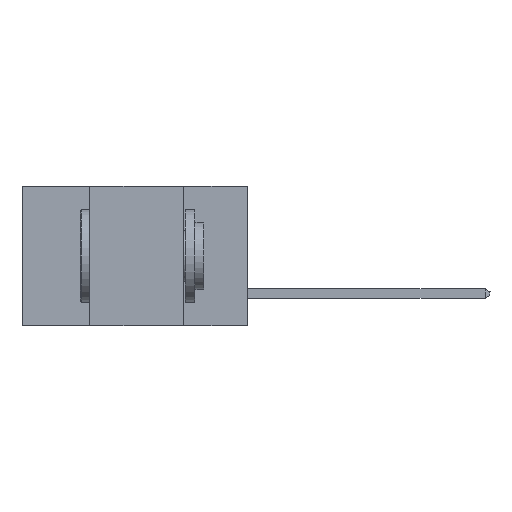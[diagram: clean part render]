
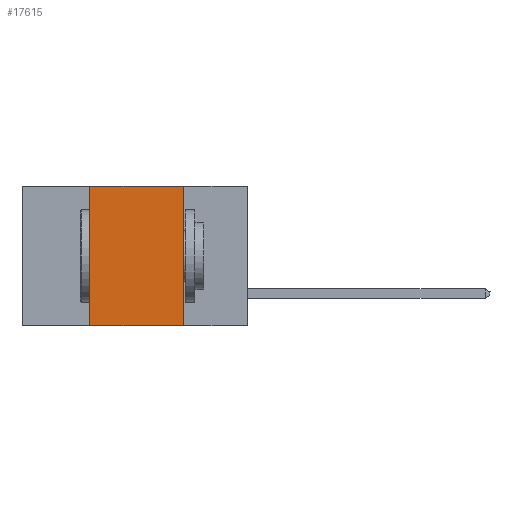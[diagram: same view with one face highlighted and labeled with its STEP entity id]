
A CAD part, left-side view. The second image highlights one B-rep face of the part: STEP entity #17615.
In plain terms, the highlighted planar face has unit normal (-1, 0, 0).
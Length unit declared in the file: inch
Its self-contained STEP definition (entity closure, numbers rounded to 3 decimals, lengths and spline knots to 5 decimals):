
#25 = EDGE_CURVE ( 'NONE', #7448, #22816, #8472, .T. ) ;
#639 = CARTESIAN_POINT ( 'NONE',  ( 0., 0.42, -0.37 ) ) ;
#665 = LINE ( 'NONE', #17799, #3531 ) ;
#713 = CARTESIAN_POINT ( 'NONE',  ( 0., 0.6, 0. ) ) ;
#909 = EDGE_CURVE ( 'NONE', #7448, #4018, #665, .T. ) ;
#1226 = AXIS2_PLACEMENT_3D ( 'NONE', #713, #13991, #21608 ) ;
#1958 = LINE ( 'NONE', #5464, #15267 ) ;
#2379 = CARTESIAN_POINT ( 'NONE',  ( 0., 0.42, -0.37 ) ) ;
#2574 = FACE_OUTER_BOUND ( 'NONE', #11931, .T. ) ;
#3152 = CARTESIAN_POINT ( 'NONE',  ( 0., 0.17, -0.37 ) ) ;
#3415 = CARTESIAN_POINT ( 'NONE',  ( 0., 0.17, 0. ) ) ;
#3531 = VECTOR ( 'NONE', #14071, 39.37008 ) ;
#4018 = VERTEX_POINT ( 'NONE', #16116 ) ;
#5464 = CARTESIAN_POINT ( 'NONE',  ( 0., 0.6, 0. ) ) ;
#7202 = VECTOR ( 'NONE', #12820, 39.37008 ) ;
#7448 = VERTEX_POINT ( 'NONE', #2379 ) ;
#7686 = CARTESIAN_POINT ( 'NONE',  ( 0., 0.42, 0. ) ) ;
#8461 = ORIENTED_EDGE ( 'NONE', *, *, #22922, .F. ) ;
#8472 = LINE ( 'NONE', #639, #16629 ) ;
#8474 = ORIENTED_EDGE ( 'NONE', *, *, #909, .T. ) ;
#11931 = EDGE_LOOP ( 'NONE', ( #13715, #8461, #13375, #8474 ) ) ;
#12175 = DIRECTION ( 'NONE',  ( 0., 0., 1. ) ) ;
#12695 = LINE ( 'NONE', #3152, #7202 ) ;
#12820 = DIRECTION ( 'NONE',  ( 0., 0., -1. ) ) ;
#13375 = ORIENTED_EDGE ( 'NONE', *, *, #25, .F. ) ;
#13715 = ORIENTED_EDGE ( 'NONE', *, *, #17788, .F. ) ;
#13991 = DIRECTION ( 'NONE',  ( 1., 0., 0. ) ) ;
#14071 = DIRECTION ( 'NONE',  ( 0., -1., 0. ) ) ;
#15267 = VECTOR ( 'NONE', #20625, 39.37008 ) ;
#16116 = CARTESIAN_POINT ( 'NONE',  ( 0., 0.17, -0.37 ) ) ;
#16376 = VERTEX_POINT ( 'NONE', #3415 ) ;
#16629 = VECTOR ( 'NONE', #12175, 39.37008 ) ;
#17615 = ADVANCED_FACE ( 'NONE', ( #2574 ), #17728, .F. ) ;
#17728 = PLANE ( 'NONE',  #1226 ) ;
#17788 = EDGE_CURVE ( 'NONE', #16376, #4018, #12695, .T. ) ;
#17799 = CARTESIAN_POINT ( 'NONE',  ( 0., 0.6, -0.37 ) ) ;
#20625 = DIRECTION ( 'NONE',  ( 0., -1., 0. ) ) ;
#21608 = DIRECTION ( 'NONE',  ( 0., 0., -1. ) ) ;
#22816 = VERTEX_POINT ( 'NONE', #7686 ) ;
#22922 = EDGE_CURVE ( 'NONE', #22816, #16376, #1958, .T. ) ;
